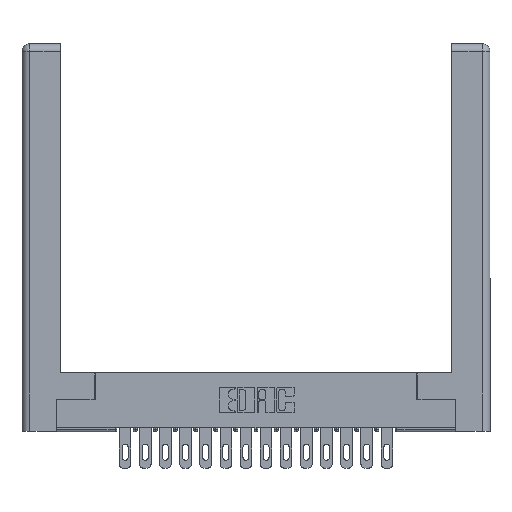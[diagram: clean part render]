
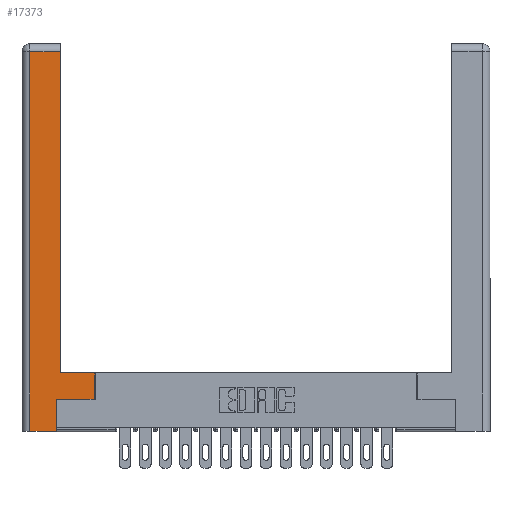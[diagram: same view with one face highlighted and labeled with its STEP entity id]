
A CAD part, top view. The second image highlights one B-rep face of the part: STEP entity #17373.
In plain terms, the highlighted planar face has unit normal (0, 0, 1).
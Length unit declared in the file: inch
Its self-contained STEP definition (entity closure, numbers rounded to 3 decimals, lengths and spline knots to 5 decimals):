
#309 = PLANE ( 'NONE',  #17065 ) ;
#569 = ORIENTED_EDGE ( 'NONE', *, *, #3196, .T. ) ;
#668 = DIRECTION ( 'NONE',  ( 0., 1., 0. ) ) ;
#750 = CARTESIAN_POINT ( 'NONE',  ( 0.0615, 0., 0. ) ) ;
#1474 = EDGE_CURVE ( 'NONE', #10946, #3421, #18686, .T. ) ;
#1818 = VERTEX_POINT ( 'NONE', #15498 ) ;
#2610 = CARTESIAN_POINT ( 'NONE',  ( 0.565, 0.245, 0. ) ) ;
#2779 = EDGE_CURVE ( 'NONE', #12342, #1818, #10920, .T. ) ;
#3196 = EDGE_CURVE ( 'NONE', #6276, #10946, #7826, .T. ) ;
#3394 = VECTOR ( 'NONE', #11789, 39.37008 ) ;
#3421 = VERTEX_POINT ( 'NONE', #3901 ) ;
#3514 = VECTOR ( 'NONE', #5836, 39.37008 ) ;
#3688 = LINE ( 'NONE', #4794, #20577 ) ;
#3901 = CARTESIAN_POINT ( 'NONE',  ( 0.565, 0.45, 0. ) ) ;
#3983 = CARTESIAN_POINT ( 'NONE',  ( 0.265, 0., 0. ) ) ;
#4409 = VERTEX_POINT ( 'NONE', #8511 ) ;
#4549 = LINE ( 'NONE', #3983, #17135 ) ;
#4717 = DIRECTION ( 'NONE',  ( -1., 0., 0. ) ) ;
#4794 = CARTESIAN_POINT ( 'NONE',  ( 0.0615, 2.94, 0. ) ) ;
#4847 = VECTOR ( 'NONE', #668, 39.37008 ) ;
#5515 = CARTESIAN_POINT ( 'NONE',  ( 0.0615, 2.94, 0. ) ) ;
#5602 = DIRECTION ( 'NONE',  ( -1., 0., 0. ) ) ;
#5664 = ORIENTED_EDGE ( 'NONE', *, *, #17887, .T. ) ;
#5780 = DIRECTION ( 'NONE',  ( 0., -1., 0. ) ) ;
#5836 = DIRECTION ( 'NONE',  ( 1., 0., 0. ) ) ;
#6276 = VERTEX_POINT ( 'NONE', #10941 ) ;
#7294 = DIRECTION ( 'NONE',  ( -1., 0., 0. ) ) ;
#7666 = ORIENTED_EDGE ( 'NONE', *, *, #20563, .T. ) ;
#7826 = LINE ( 'NONE', #14911, #3514 ) ;
#8201 = VECTOR ( 'NONE', #15023, 39.37008 ) ;
#8511 = CARTESIAN_POINT ( 'NONE',  ( 0.295, 2.94, 0. ) ) ;
#8679 = VERTEX_POINT ( 'NONE', #11540 ) ;
#9339 = ORIENTED_EDGE ( 'NONE', *, *, #1474, .T. ) ;
#9432 = EDGE_LOOP ( 'NONE', ( #10225, #12963, #15799, #7666, #5664, #569, #9339, #14546 ) ) ;
#9502 = LINE ( 'NONE', #16707, #3394 ) ;
#10225 = ORIENTED_EDGE ( 'NONE', *, *, #19329, .T. ) ;
#10920 = LINE ( 'NONE', #750, #14526 ) ;
#10941 = CARTESIAN_POINT ( 'NONE',  ( 0.265, 0.245, 0. ) ) ;
#10946 = VERTEX_POINT ( 'NONE', #2610 ) ;
#11069 = FACE_OUTER_BOUND ( 'NONE', #9432, .T. ) ;
#11540 = CARTESIAN_POINT ( 'NONE',  ( 0.265, 0., 0. ) ) ;
#11789 = DIRECTION ( 'NONE',  ( 0., 1., 0. ) ) ;
#12342 = VERTEX_POINT ( 'NONE', #5515 ) ;
#12414 = EDGE_CURVE ( 'NONE', #3421, #15632, #16177, .T. ) ;
#12791 = VECTOR ( 'NONE', #7294, 39.37008 ) ;
#12963 = ORIENTED_EDGE ( 'NONE', *, *, #17534, .T. ) ;
#14526 = VECTOR ( 'NONE', #5780, 39.37008 ) ;
#14546 = ORIENTED_EDGE ( 'NONE', *, *, #12414, .T. ) ;
#14911 = CARTESIAN_POINT ( 'NONE',  ( 0.565, 0.245, 0. ) ) ;
#15023 = DIRECTION ( 'NONE',  ( 0., 1., 0. ) ) ;
#15454 = CARTESIAN_POINT ( 'NONE',  ( 0.565, 0.45, 0. ) ) ;
#15498 = CARTESIAN_POINT ( 'NONE',  ( 0.0615, 0., 0. ) ) ;
#15632 = VERTEX_POINT ( 'NONE', #15722 ) ;
#15722 = CARTESIAN_POINT ( 'NONE',  ( 0.295, 0.45, 0. ) ) ;
#15799 = ORIENTED_EDGE ( 'NONE', *, *, #2779, .T. ) ;
#16177 = LINE ( 'NONE', #17134, #12791 ) ;
#16707 = CARTESIAN_POINT ( 'NONE',  ( 0.265, 0.245, 0. ) ) ;
#16901 = DIRECTION ( 'NONE',  ( 1., 0., 0. ) ) ;
#17065 = AXIS2_PLACEMENT_3D ( 'NONE', #20084, #18646, #5602 ) ;
#17134 = CARTESIAN_POINT ( 'NONE',  ( 0.295, 0.45, 0. ) ) ;
#17135 = VECTOR ( 'NONE', #16901, 39.37008 ) ;
#17191 = LINE ( 'NONE', #18257, #8201 ) ;
#17373 = ADVANCED_FACE ( 'NONE', ( #11069 ), #309, .F. ) ;
#17534 = EDGE_CURVE ( 'NONE', #4409, #12342, #3688, .T. ) ;
#17887 = EDGE_CURVE ( 'NONE', #8679, #6276, #9502, .T. ) ;
#18257 = CARTESIAN_POINT ( 'NONE',  ( 0.295, 3., 0. ) ) ;
#18646 = DIRECTION ( 'NONE',  ( 0., 0., -1. ) ) ;
#18686 = LINE ( 'NONE', #15454, #4847 ) ;
#19329 = EDGE_CURVE ( 'NONE', #15632, #4409, #17191, .T. ) ;
#20084 = CARTESIAN_POINT ( 'NONE',  ( 0., 0., 0. ) ) ;
#20563 = EDGE_CURVE ( 'NONE', #1818, #8679, #4549, .T. ) ;
#20577 = VECTOR ( 'NONE', #4717, 39.37008 ) ;
